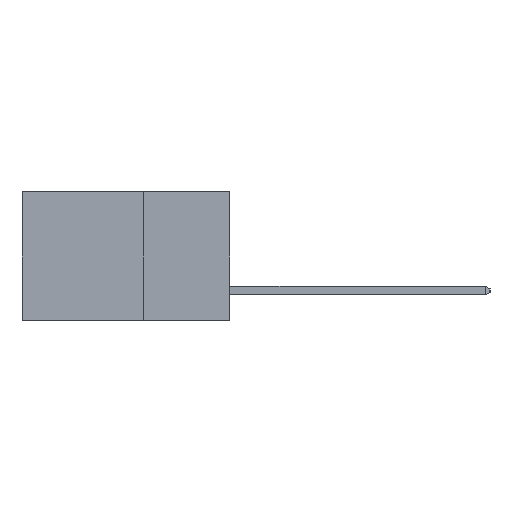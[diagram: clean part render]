
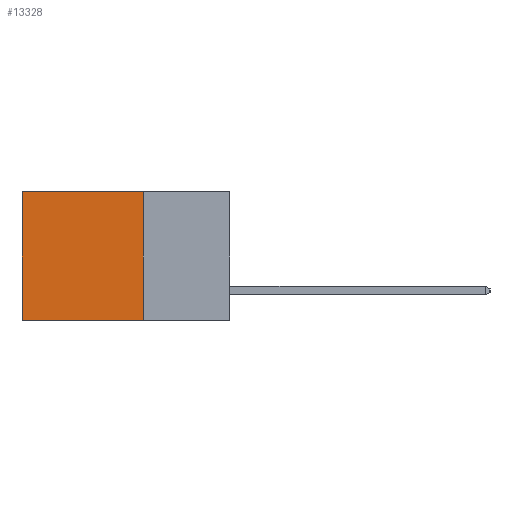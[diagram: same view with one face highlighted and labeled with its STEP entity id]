
A CAD part, left-side view. The second image highlights one B-rep face of the part: STEP entity #13328.
In plain terms, the highlighted planar face has unit normal (-1, 0, 0).
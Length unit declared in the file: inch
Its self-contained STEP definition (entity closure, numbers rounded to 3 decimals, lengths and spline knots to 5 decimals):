
#342 = EDGE_CURVE ( 'NONE', #16509, #5027, #5518, .T. ) ;
#1419 = EDGE_CURVE ( 'NONE', #3869, #5027, #16521, .T. ) ;
#2066 = VECTOR ( 'NONE', #10808, 39.37008 ) ;
#2586 = VECTOR ( 'NONE', #15742, 39.37008 ) ;
#2618 = AXIS2_PLACEMENT_3D ( 'NONE', #3913, #15330, #7780 ) ;
#2735 = ORIENTED_EDGE ( 'NONE', *, *, #8760, .T. ) ;
#3319 = CARTESIAN_POINT ( 'NONE',  ( 0.2615, 0.6, -0.37 ) ) ;
#3431 = VECTOR ( 'NONE', #5335, 39.37008 ) ;
#3482 = FACE_OUTER_BOUND ( 'NONE', #10032, .T. ) ;
#3869 = VERTEX_POINT ( 'NONE', #7482 ) ;
#3913 = CARTESIAN_POINT ( 'NONE',  ( 0.2615, 0.25, -0.37 ) ) ;
#4293 = CARTESIAN_POINT ( 'NONE',  ( 0.2615, 0.6, -0.37 ) ) ;
#5027 = VERTEX_POINT ( 'NONE', #3319 ) ;
#5335 = DIRECTION ( 'NONE',  ( 0., 1., 0. ) ) ;
#5518 = LINE ( 'NONE', #4293, #2066 ) ;
#7482 = CARTESIAN_POINT ( 'NONE',  ( 0.2615, 0.25, -0.37 ) ) ;
#7780 = DIRECTION ( 'NONE',  ( 0., 0., -1. ) ) ;
#8760 = EDGE_CURVE ( 'NONE', #11613, #16509, #16111, .T. ) ;
#9050 = CARTESIAN_POINT ( 'NONE',  ( 0.2615, 0.25, 0. ) ) ;
#9834 = LINE ( 'NONE', #10717, #2586 ) ;
#10032 = EDGE_LOOP ( 'NONE', ( #12646, #13842, #12603, #2735 ) ) ;
#10717 = CARTESIAN_POINT ( 'NONE',  ( 0.2615, 0.25, -0.37 ) ) ;
#10808 = DIRECTION ( 'NONE',  ( 0., 0., -1. ) ) ;
#11613 = VERTEX_POINT ( 'NONE', #9050 ) ;
#12603 = ORIENTED_EDGE ( 'NONE', *, *, #15992, .F. ) ;
#12646 = ORIENTED_EDGE ( 'NONE', *, *, #342, .T. ) ;
#13257 = VECTOR ( 'NONE', #15116, 39.37008 ) ;
#13328 = ADVANCED_FACE ( 'NONE', ( #3482 ), #14075, .F. ) ;
#13634 = CARTESIAN_POINT ( 'NONE',  ( 0.2615, 0.6, 0. ) ) ;
#13842 = ORIENTED_EDGE ( 'NONE', *, *, #1419, .F. ) ;
#14075 = PLANE ( 'NONE',  #2618 ) ;
#14218 = CARTESIAN_POINT ( 'NONE',  ( 0.2615, 0.25, 0. ) ) ;
#15116 = DIRECTION ( 'NONE',  ( 0., 1., 0. ) ) ;
#15330 = DIRECTION ( 'NONE',  ( 1., 0., 0. ) ) ;
#15742 = DIRECTION ( 'NONE',  ( 0., 0., -1. ) ) ;
#15880 = CARTESIAN_POINT ( 'NONE',  ( 0.2615, 0.25, -0.37 ) ) ;
#15992 = EDGE_CURVE ( 'NONE', #11613, #3869, #9834, .T. ) ;
#16111 = LINE ( 'NONE', #14218, #3431 ) ;
#16509 = VERTEX_POINT ( 'NONE', #13634 ) ;
#16521 = LINE ( 'NONE', #15880, #13257 ) ;
